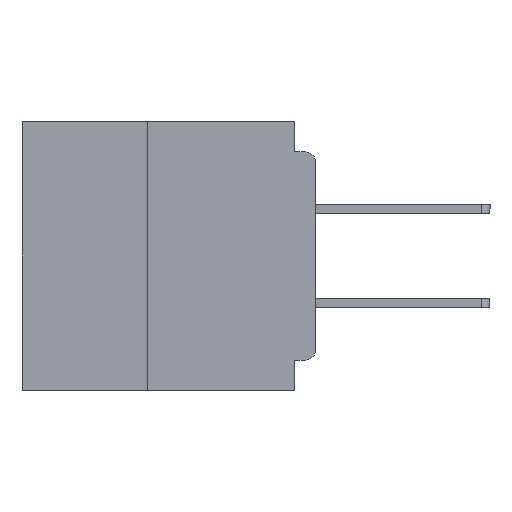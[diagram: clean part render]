
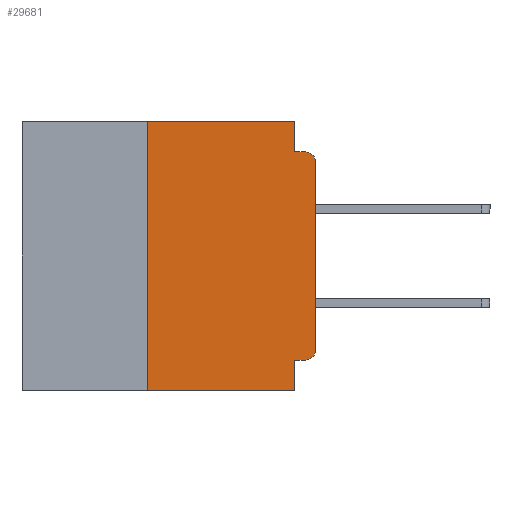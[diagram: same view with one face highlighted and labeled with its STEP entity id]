
A CAD part, left-side view. The second image highlights one B-rep face of the part: STEP entity #29681.
In plain terms, the highlighted planar face has unit normal (-1, 0, 0).
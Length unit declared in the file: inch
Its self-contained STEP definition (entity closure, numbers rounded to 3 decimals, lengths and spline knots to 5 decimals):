
#26 = DIRECTION ( 'NONE',  ( -1., 0., 0. ) ) ;
#1789 = VERTEX_POINT ( 'NONE', #25245 ) ;
#2127 = AXIS2_PLACEMENT_3D ( 'NONE', #29869, #38877, #20851 ) ;
#2536 = EDGE_CURVE ( 'NONE', #9029, #26175, #18857, .T. ) ;
#2605 = VERTEX_POINT ( 'NONE', #4865 ) ;
#2806 = CARTESIAN_POINT ( 'NONE',  ( 0., 0.25, -0.4 ) ) ;
#2822 = ORIENTED_EDGE ( 'NONE', *, *, #33865, .F. ) ;
#3166 = CARTESIAN_POINT ( 'NONE',  ( 0., 0.031, -0.045 ) ) ;
#3311 = CARTESIAN_POINT ( 'NONE',  ( 0., 0.015, -0.06 ) ) ;
#3504 = DIRECTION ( 'NONE',  ( 0., 0., -1. ) ) ;
#3868 = VECTOR ( 'NONE', #7020, 39.37008 ) ;
#4797 = ORIENTED_EDGE ( 'NONE', *, *, #2536, .T. ) ;
#4865 = CARTESIAN_POINT ( 'NONE',  ( 0., 0.015, -0.355 ) ) ;
#5202 = EDGE_CURVE ( 'NONE', #2605, #10138, #15942, .T. ) ;
#5599 = VERTEX_POINT ( 'NONE', #6378 ) ;
#6139 = VERTEX_POINT ( 'NONE', #2806 ) ;
#6378 = CARTESIAN_POINT ( 'NONE',  ( 0., 0.015, -0.045 ) ) ;
#6433 = DIRECTION ( 'NONE',  ( 0., 0., -1. ) ) ;
#6475 = CARTESIAN_POINT ( 'NONE',  ( 0., 0.031, -0.355 ) ) ;
#6785 = LINE ( 'NONE', #31219, #3868 ) ;
#7020 = DIRECTION ( 'NONE',  ( 0., 0., -1. ) ) ;
#7041 = VECTOR ( 'NONE', #39150, 39.37008 ) ;
#7155 = ORIENTED_EDGE ( 'NONE', *, *, #8663, .F. ) ;
#7525 = CARTESIAN_POINT ( 'NONE',  ( 0., 0.031, -0.4 ) ) ;
#8599 = EDGE_CURVE ( 'NONE', #1789, #16131, #14209, .T. ) ;
#8663 = EDGE_CURVE ( 'NONE', #24847, #5599, #22322, .T. ) ;
#9029 = VERTEX_POINT ( 'NONE', #37146 ) ;
#9554 = CARTESIAN_POINT ( 'NONE',  ( 0., 0.031, -0.4 ) ) ;
#10138 = VERTEX_POINT ( 'NONE', #6475 ) ;
#10367 = CARTESIAN_POINT ( 'NONE',  ( 0., 0.437, -0.4 ) ) ;
#10627 = CARTESIAN_POINT ( 'NONE',  ( 0., 0., 0. ) ) ;
#10744 = VECTOR ( 'NONE', #10763, 39.37008 ) ;
#10763 = DIRECTION ( 'NONE',  ( 0., 0., 1. ) ) ;
#13231 = VECTOR ( 'NONE', #35224, 39.37008 ) ;
#13722 = VERTEX_POINT ( 'NONE', #7525 ) ;
#14209 = LINE ( 'NONE', #32221, #13231 ) ;
#15942 = LINE ( 'NONE', #37789, #23049 ) ;
#16131 = VERTEX_POINT ( 'NONE', #33883 ) ;
#16250 = ORIENTED_EDGE ( 'NONE', *, *, #25512, .F. ) ;
#17083 = DIRECTION ( 'NONE',  ( 0., -1., 0. ) ) ;
#17403 = LINE ( 'NONE', #10367, #20700 ) ;
#18443 = CARTESIAN_POINT ( 'NONE',  ( 0., 0.015, -0.34 ) ) ;
#18857 = LINE ( 'NONE', #10627, #10744 ) ;
#20700 = VECTOR ( 'NONE', #22742, 39.37008 ) ;
#20851 = DIRECTION ( 'NONE',  ( 0., 0., -1. ) ) ;
#21476 = DIRECTION ( 'NONE',  ( 0., 0., -1. ) ) ;
#22322 = LINE ( 'NONE', #35184, #39266 ) ;
#22742 = DIRECTION ( 'NONE',  ( 0., -1., 0. ) ) ;
#22775 = DIRECTION ( 'NONE',  ( 0., 1., 0. ) ) ;
#23049 = VECTOR ( 'NONE', #22775, 39.37008 ) ;
#23288 = AXIS2_PLACEMENT_3D ( 'NONE', #18443, #26, #21476 ) ;
#23753 = EDGE_CURVE ( 'NONE', #6139, #13722, #17403, .T. ) ;
#23980 = EDGE_LOOP ( 'NONE', ( #4797, #30478, #7155, #16250, #32358, #25275, #34221, #2822, #27181, #29079 ) ) ;
#24179 = CARTESIAN_POINT ( 'NONE',  ( 0., 0.25, -0.4 ) ) ;
#24210 = LINE ( 'NONE', #24179, #7041 ) ;
#24676 = DIRECTION ( 'NONE',  ( -1., 0., 0. ) ) ;
#24847 = VERTEX_POINT ( 'NONE', #3166 ) ;
#25245 = CARTESIAN_POINT ( 'NONE',  ( 0., 0.25, 0. ) ) ;
#25275 = ORIENTED_EDGE ( 'NONE', *, *, #27787, .F. ) ;
#25512 = EDGE_CURVE ( 'NONE', #16131, #24847, #6785, .T. ) ;
#26175 = VERTEX_POINT ( 'NONE', #37848 ) ;
#26568 = EDGE_CURVE ( 'NONE', #26175, #5599, #36551, .T. ) ;
#26877 = AXIS2_PLACEMENT_3D ( 'NONE', #3311, #24676, #6433 ) ;
#27181 = ORIENTED_EDGE ( 'NONE', *, *, #5202, .F. ) ;
#27201 = CIRCLE ( 'NONE', #23288, 0.015 ) ;
#27787 = EDGE_CURVE ( 'NONE', #6139, #1789, #24210, .T. ) ;
#27971 = FACE_OUTER_BOUND ( 'NONE', #23980, .T. ) ;
#28506 = VECTOR ( 'NONE', #3504, 39.37008 ) ;
#29079 = ORIENTED_EDGE ( 'NONE', *, *, #37355, .T. ) ;
#29482 = LINE ( 'NONE', #9554, #28506 ) ;
#29681 = ADVANCED_FACE ( 'NONE', ( #27971 ), #35877, .F. ) ;
#29869 = CARTESIAN_POINT ( 'NONE',  ( 0., 0.437, 0. ) ) ;
#30478 = ORIENTED_EDGE ( 'NONE', *, *, #26568, .T. ) ;
#31219 = CARTESIAN_POINT ( 'NONE',  ( 0., 0.031, 0. ) ) ;
#32221 = CARTESIAN_POINT ( 'NONE',  ( 0., 0.437, 0. ) ) ;
#32358 = ORIENTED_EDGE ( 'NONE', *, *, #8599, .F. ) ;
#33865 = EDGE_CURVE ( 'NONE', #10138, #13722, #29482, .T. ) ;
#33883 = CARTESIAN_POINT ( 'NONE',  ( 0., 0.031, 0. ) ) ;
#34221 = ORIENTED_EDGE ( 'NONE', *, *, #23753, .T. ) ;
#35184 = CARTESIAN_POINT ( 'NONE',  ( 0., 0., -0.045 ) ) ;
#35224 = DIRECTION ( 'NONE',  ( 0., -1., 0. ) ) ;
#35877 = PLANE ( 'NONE',  #2127 ) ;
#36551 = CIRCLE ( 'NONE', #26877, 0.015 ) ;
#37146 = CARTESIAN_POINT ( 'NONE',  ( 0., 0., -0.34 ) ) ;
#37355 = EDGE_CURVE ( 'NONE', #2605, #9029, #27201, .T. ) ;
#37789 = CARTESIAN_POINT ( 'NONE',  ( 0., 0., -0.355 ) ) ;
#37848 = CARTESIAN_POINT ( 'NONE',  ( 0., 0., -0.06 ) ) ;
#38877 = DIRECTION ( 'NONE',  ( 1., 0., 0. ) ) ;
#39150 = DIRECTION ( 'NONE',  ( 0., 0., 1. ) ) ;
#39266 = VECTOR ( 'NONE', #17083, 39.37008 ) ;
